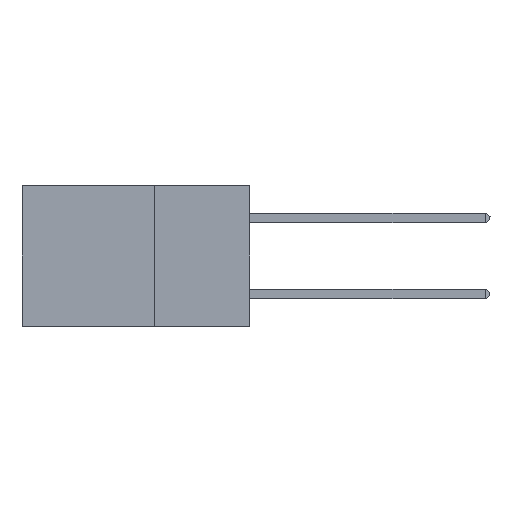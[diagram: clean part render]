
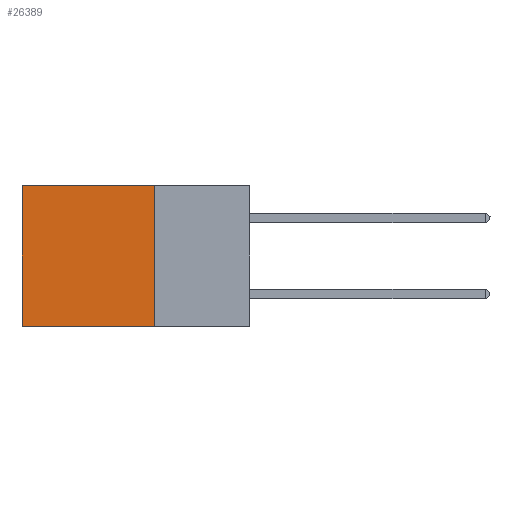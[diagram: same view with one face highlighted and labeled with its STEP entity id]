
A CAD part, left-side view. The second image highlights one B-rep face of the part: STEP entity #26389.
In plain terms, the highlighted planar face has unit normal (-1, 0, 0).
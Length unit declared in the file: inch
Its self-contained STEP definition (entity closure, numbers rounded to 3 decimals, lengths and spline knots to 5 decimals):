
#506 = ORIENTED_EDGE ( 'NONE', *, *, #20232, .F. ) ;
#755 = DIRECTION ( 'NONE',  ( 0., 0., -1. ) ) ;
#1302 = CARTESIAN_POINT ( 'NONE',  ( 0.2875, 0.6, -0.37 ) ) ;
#1388 = CARTESIAN_POINT ( 'NONE',  ( 0.2875, 0.6, 0. ) ) ;
#4187 = DIRECTION ( 'NONE',  ( 1., 0., 0. ) ) ;
#5439 = VECTOR ( 'NONE', #25495, 39.37008 ) ;
#7006 = EDGE_CURVE ( 'NONE', #35527, #44056, #17701, .T. ) ;
#7644 = ORIENTED_EDGE ( 'NONE', *, *, #27296, .F. ) ;
#7648 = DIRECTION ( 'NONE',  ( 0., 1., 0. ) ) ;
#7686 = LINE ( 'NONE', #22051, #26301 ) ;
#9963 = LINE ( 'NONE', #20453, #27363 ) ;
#11349 = CARTESIAN_POINT ( 'NONE',  ( 0.2875, 0.25, -0.37 ) ) ;
#11785 = CARTESIAN_POINT ( 'NONE',  ( 0.2875, 0.25, 0. ) ) ;
#12254 = VERTEX_POINT ( 'NONE', #16191 ) ;
#12619 = VERTEX_POINT ( 'NONE', #1302 ) ;
#14494 = CARTESIAN_POINT ( 'NONE',  ( 0.2875, 0.25, 0. ) ) ;
#16191 = CARTESIAN_POINT ( 'NONE',  ( 0.2875, 0.25, -0.37 ) ) ;
#17701 = LINE ( 'NONE', #31847, #26802 ) ;
#20232 = EDGE_CURVE ( 'NONE', #35527, #12254, #9963, .T. ) ;
#20453 = CARTESIAN_POINT ( 'NONE',  ( 0.2875, 0.25, 0. ) ) ;
#21547 = PLANE ( 'NONE',  #34159 ) ;
#22051 = CARTESIAN_POINT ( 'NONE',  ( 0.2875, 0.6, 0. ) ) ;
#25209 = FACE_OUTER_BOUND ( 'NONE', #26844, .T. ) ;
#25495 = DIRECTION ( 'NONE',  ( 0., 1., 0. ) ) ;
#26301 = VECTOR ( 'NONE', #32802, 39.37008 ) ;
#26389 = ADVANCED_FACE ( 'NONE', ( #25209 ), #21547, .F. ) ;
#26802 = VECTOR ( 'NONE', #7648, 39.37008 ) ;
#26844 = EDGE_LOOP ( 'NONE', ( #38932, #7644, #506, #30393 ) ) ;
#27296 = EDGE_CURVE ( 'NONE', #12254, #12619, #38725, .T. ) ;
#27363 = VECTOR ( 'NONE', #34388, 39.37008 ) ;
#30393 = ORIENTED_EDGE ( 'NONE', *, *, #7006, .T. ) ;
#31847 = CARTESIAN_POINT ( 'NONE',  ( 0.2875, 0.25, 0. ) ) ;
#32802 = DIRECTION ( 'NONE',  ( 0., 0., -1. ) ) ;
#34159 = AXIS2_PLACEMENT_3D ( 'NONE', #14494, #4187, #755 ) ;
#34388 = DIRECTION ( 'NONE',  ( 0., 0., -1. ) ) ;
#35527 = VERTEX_POINT ( 'NONE', #11785 ) ;
#38725 = LINE ( 'NONE', #11349, #5439 ) ;
#38932 = ORIENTED_EDGE ( 'NONE', *, *, #44369, .T. ) ;
#44056 = VERTEX_POINT ( 'NONE', #1388 ) ;
#44369 = EDGE_CURVE ( 'NONE', #44056, #12619, #7686, .T. ) ;
